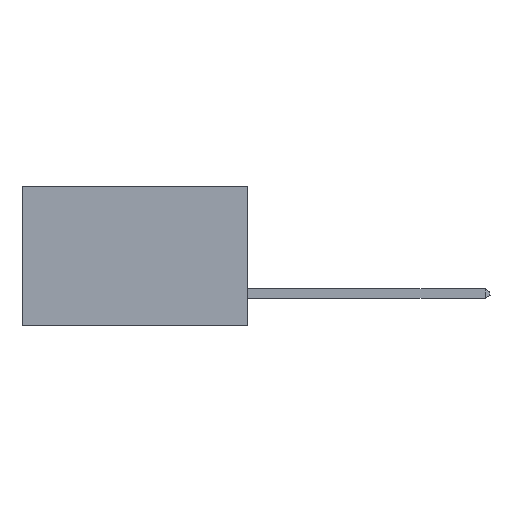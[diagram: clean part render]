
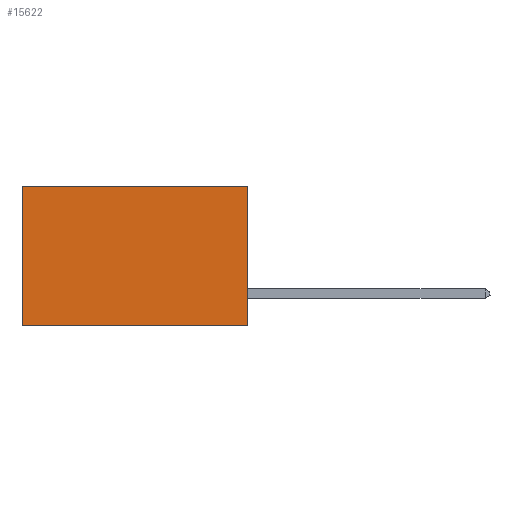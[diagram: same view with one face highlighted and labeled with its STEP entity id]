
A CAD part, left-side view. The second image highlights one B-rep face of the part: STEP entity #15622.
In plain terms, the highlighted planar face has unit normal (-1, 0, 0).
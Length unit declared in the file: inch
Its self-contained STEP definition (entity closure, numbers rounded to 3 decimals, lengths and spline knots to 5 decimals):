
#276 = DIRECTION ( 'NONE',  ( 1., 0., 0. ) ) ;
#1438 = DIRECTION ( 'NONE',  ( 0., 0., -1. ) ) ;
#1631 = VECTOR ( 'NONE', #7883, 39.37008 ) ;
#2324 = CARTESIAN_POINT ( 'NONE',  ( 0.298, 0.6, 0. ) ) ;
#2792 = DIRECTION ( 'NONE',  ( 0., 1., 0. ) ) ;
#3300 = CARTESIAN_POINT ( 'NONE',  ( 0.298, 0.6, -0.37 ) ) ;
#3652 = CARTESIAN_POINT ( 'NONE',  ( 0.298, 0., 0. ) ) ;
#3890 = PLANE ( 'NONE',  #11971 ) ;
#4409 = CARTESIAN_POINT ( 'NONE',  ( 0.298, 0.6, 0. ) ) ;
#6401 = LINE ( 'NONE', #4409, #1631 ) ;
#7014 = CARTESIAN_POINT ( 'NONE',  ( 0.298, 0., 0. ) ) ;
#7883 = DIRECTION ( 'NONE',  ( 0., 0., -1. ) ) ;
#8282 = CARTESIAN_POINT ( 'NONE',  ( 0.298, 0., -0.37 ) ) ;
#8401 = ORIENTED_EDGE ( 'NONE', *, *, #11152, .F. ) ;
#8639 = ORIENTED_EDGE ( 'NONE', *, *, #17686, .T. ) ;
#8654 = VECTOR ( 'NONE', #1438, 39.37008 ) ;
#9443 = VERTEX_POINT ( 'NONE', #3652 ) ;
#10410 = EDGE_CURVE ( 'NONE', #11907, #14353, #17581, .T. ) ;
#11152 = EDGE_CURVE ( 'NONE', #9443, #11907, #13548, .T. ) ;
#11474 = CARTESIAN_POINT ( 'NONE',  ( 0.298, 0., 0. ) ) ;
#11907 = VERTEX_POINT ( 'NONE', #23443 ) ;
#11971 = AXIS2_PLACEMENT_3D ( 'NONE', #11474, #276, #20556 ) ;
#12670 = ORIENTED_EDGE ( 'NONE', *, *, #10410, .F. ) ;
#13397 = CARTESIAN_POINT ( 'NONE',  ( 0.298, 0., 0. ) ) ;
#13548 = LINE ( 'NONE', #7014, #8654 ) ;
#13876 = VECTOR ( 'NONE', #2792, 39.37008 ) ;
#14353 = VERTEX_POINT ( 'NONE', #3300 ) ;
#15622 = ADVANCED_FACE ( 'NONE', ( #23233 ), #3890, .F. ) ;
#16163 = EDGE_LOOP ( 'NONE', ( #23081, #12670, #8401, #8639 ) ) ;
#17581 = LINE ( 'NONE', #8282, #13876 ) ;
#17686 = EDGE_CURVE ( 'NONE', #9443, #18129, #22805, .T. ) ;
#18129 = VERTEX_POINT ( 'NONE', #2324 ) ;
#19450 = EDGE_CURVE ( 'NONE', #18129, #14353, #6401, .T. ) ;
#20556 = DIRECTION ( 'NONE',  ( 0., 0., -1. ) ) ;
#22362 = DIRECTION ( 'NONE',  ( 0., 1., 0. ) ) ;
#22805 = LINE ( 'NONE', #13397, #23117 ) ;
#23081 = ORIENTED_EDGE ( 'NONE', *, *, #19450, .T. ) ;
#23117 = VECTOR ( 'NONE', #22362, 39.37008 ) ;
#23233 = FACE_OUTER_BOUND ( 'NONE', #16163, .T. ) ;
#23443 = CARTESIAN_POINT ( 'NONE',  ( 0.298, 0., -0.37 ) ) ;
